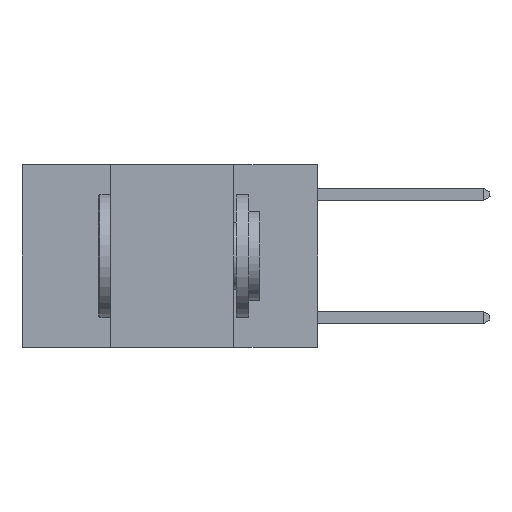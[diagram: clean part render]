
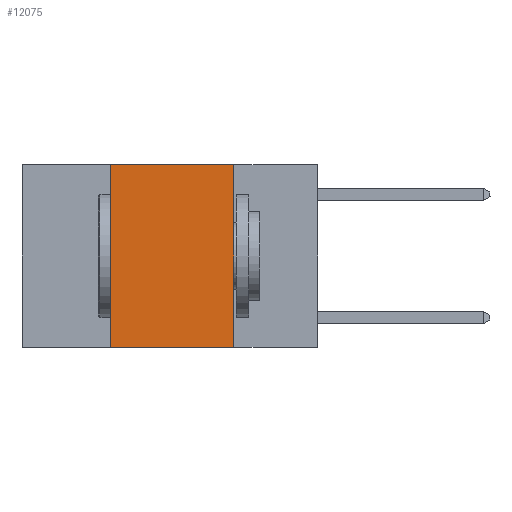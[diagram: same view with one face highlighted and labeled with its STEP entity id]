
A CAD part, left-side view. The second image highlights one B-rep face of the part: STEP entity #12075.
In plain terms, the highlighted planar face has unit normal (-1, 0, 0).
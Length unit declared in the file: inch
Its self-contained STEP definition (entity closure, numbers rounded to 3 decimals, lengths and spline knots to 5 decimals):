
#273 = PLANE ( 'NONE',  #1391 ) ;
#1015 = FACE_OUTER_BOUND ( 'NONE', #2577, .T. ) ;
#1391 = AXIS2_PLACEMENT_3D ( 'NONE', #5242, #3278, #10173 ) ;
#2018 = ORIENTED_EDGE ( 'NONE', *, *, #6845, .F. ) ;
#2400 = CARTESIAN_POINT ( 'NONE',  ( 0., 0.6, -0.37 ) ) ;
#2577 = EDGE_LOOP ( 'NONE', ( #2018, #9502, #6926, #4294 ) ) ;
#2623 = DIRECTION ( 'NONE',  ( 0., -1., 0. ) ) ;
#2735 = CARTESIAN_POINT ( 'NONE',  ( 0., 0.42, -0.37 ) ) ;
#3278 = DIRECTION ( 'NONE',  ( 1., 0., 0. ) ) ;
#3526 = LINE ( 'NONE', #12342, #8395 ) ;
#3706 = CARTESIAN_POINT ( 'NONE',  ( 0., 0.17, 0. ) ) ;
#3862 = EDGE_CURVE ( 'NONE', #11230, #11517, #3526, .T. ) ;
#4062 = CARTESIAN_POINT ( 'NONE',  ( 0., 0.17, 0. ) ) ;
#4294 = ORIENTED_EDGE ( 'NONE', *, *, #7484, .T. ) ;
#4593 = DIRECTION ( 'NONE',  ( 0., 0., 1. ) ) ;
#4766 = VECTOR ( 'NONE', #5415, 39.37008 ) ;
#5242 = CARTESIAN_POINT ( 'NONE',  ( 0., 0.6, 0. ) ) ;
#5406 = VECTOR ( 'NONE', #5749, 39.37008 ) ;
#5415 = DIRECTION ( 'NONE',  ( 0., -1., 0. ) ) ;
#5580 = CARTESIAN_POINT ( 'NONE',  ( 0., 0.17, -0.37 ) ) ;
#5749 = DIRECTION ( 'NONE',  ( 0., 0., -1. ) ) ;
#6675 = VERTEX_POINT ( 'NONE', #5580 ) ;
#6845 = EDGE_CURVE ( 'NONE', #11420, #6675, #7932, .T. ) ;
#6926 = ORIENTED_EDGE ( 'NONE', *, *, #3862, .F. ) ;
#7484 = EDGE_CURVE ( 'NONE', #11230, #6675, #7637, .T. ) ;
#7631 = EDGE_CURVE ( 'NONE', #11517, #11420, #11360, .T. ) ;
#7637 = LINE ( 'NONE', #2400, #4766 ) ;
#7932 = LINE ( 'NONE', #3706, #5406 ) ;
#8395 = VECTOR ( 'NONE', #4593, 39.37008 ) ;
#9502 = ORIENTED_EDGE ( 'NONE', *, *, #7631, .F. ) ;
#10173 = DIRECTION ( 'NONE',  ( 0., 0., -1. ) ) ;
#11056 = VECTOR ( 'NONE', #2623, 39.37008 ) ;
#11127 = CARTESIAN_POINT ( 'NONE',  ( 0., 0.42, 0. ) ) ;
#11230 = VERTEX_POINT ( 'NONE', #2735 ) ;
#11360 = LINE ( 'NONE', #12319, #11056 ) ;
#11420 = VERTEX_POINT ( 'NONE', #4062 ) ;
#11517 = VERTEX_POINT ( 'NONE', #11127 ) ;
#12075 = ADVANCED_FACE ( 'NONE', ( #1015 ), #273, .F. ) ;
#12319 = CARTESIAN_POINT ( 'NONE',  ( 0., 0.6, 0. ) ) ;
#12342 = CARTESIAN_POINT ( 'NONE',  ( 0., 0.42, 0. ) ) ;
